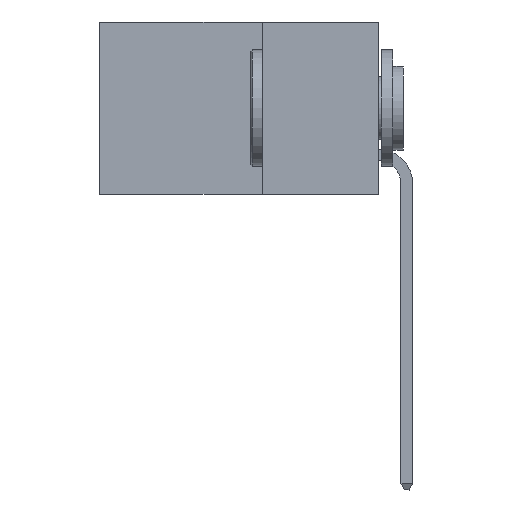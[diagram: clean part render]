
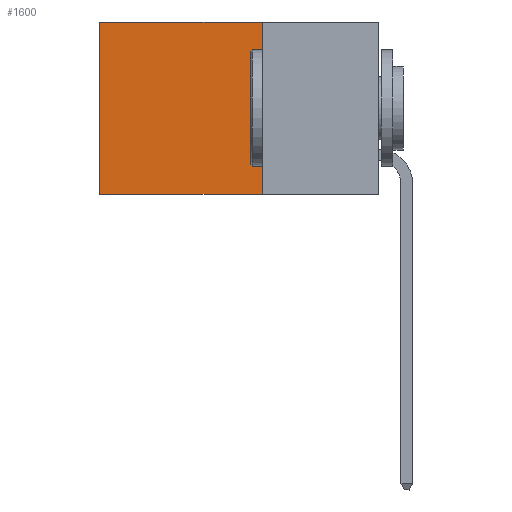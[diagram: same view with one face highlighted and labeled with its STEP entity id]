
A CAD part, left-side view. The second image highlights one B-rep face of the part: STEP entity #1600.
In plain terms, the highlighted planar face has unit normal (-1, 0, 0).
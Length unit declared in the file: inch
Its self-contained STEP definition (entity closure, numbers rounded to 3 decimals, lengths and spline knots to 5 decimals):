
#250 = CARTESIAN_POINT ( 'NONE',  ( 0.298, 0.25, 0. ) ) ;
#431 = AXIS2_PLACEMENT_3D ( 'NONE', #1900, #26840, #19964 ) ;
#1600 = ADVANCED_FACE ( 'NONE', ( #22351 ), #2191, .F. ) ;
#1900 = CARTESIAN_POINT ( 'NONE',  ( 0.298, 0.25, 0. ) ) ;
#2105 = VECTOR ( 'NONE', #18477, 39.37008 ) ;
#2172 = CARTESIAN_POINT ( 'NONE',  ( 0.298, 0.6, 0. ) ) ;
#2191 = PLANE ( 'NONE',  #431 ) ;
#3347 = ORIENTED_EDGE ( 'NONE', *, *, #16645, .F. ) ;
#3802 = CARTESIAN_POINT ( 'NONE',  ( 0.298, 0.25, -0.37 ) ) ;
#3973 = EDGE_CURVE ( 'NONE', #8858, #10029, #18820, .T. ) ;
#4275 = VECTOR ( 'NONE', #25693, 39.37008 ) ;
#5141 = ORIENTED_EDGE ( 'NONE', *, *, #5374, .F. ) ;
#5374 = EDGE_CURVE ( 'NONE', #27201, #7187, #15088, .T. ) ;
#5872 = LINE ( 'NONE', #3802, #24953 ) ;
#6548 = DIRECTION ( 'NONE',  ( 0., 0., -1. ) ) ;
#7187 = VERTEX_POINT ( 'NONE', #27425 ) ;
#7457 = CARTESIAN_POINT ( 'NONE',  ( 0.298, 0.6, 0. ) ) ;
#8858 = VERTEX_POINT ( 'NONE', #2172 ) ;
#9078 = LINE ( 'NONE', #250, #2105 ) ;
#10029 = VERTEX_POINT ( 'NONE', #20120 ) ;
#13866 = EDGE_LOOP ( 'NONE', ( #25352, #3347, #5141, #16098 ) ) ;
#15088 = LINE ( 'NONE', #17914, #23397 ) ;
#15148 = DIRECTION ( 'NONE',  ( 0., 1., 0. ) ) ;
#16063 = EDGE_CURVE ( 'NONE', #27201, #8858, #9078, .T. ) ;
#16098 = ORIENTED_EDGE ( 'NONE', *, *, #16063, .T. ) ;
#16645 = EDGE_CURVE ( 'NONE', #7187, #10029, #5872, .T. ) ;
#17914 = CARTESIAN_POINT ( 'NONE',  ( 0.298, 0.25, 0. ) ) ;
#18477 = DIRECTION ( 'NONE',  ( 0., 1., 0. ) ) ;
#18820 = LINE ( 'NONE', #7457, #4275 ) ;
#19019 = CARTESIAN_POINT ( 'NONE',  ( 0.298, 0.25, 0. ) ) ;
#19964 = DIRECTION ( 'NONE',  ( 0., 0., -1. ) ) ;
#20120 = CARTESIAN_POINT ( 'NONE',  ( 0.298, 0.6, -0.37 ) ) ;
#22351 = FACE_OUTER_BOUND ( 'NONE', #13866, .T. ) ;
#23397 = VECTOR ( 'NONE', #6548, 39.37008 ) ;
#24953 = VECTOR ( 'NONE', #15148, 39.37008 ) ;
#25352 = ORIENTED_EDGE ( 'NONE', *, *, #3973, .T. ) ;
#25693 = DIRECTION ( 'NONE',  ( 0., 0., -1. ) ) ;
#26840 = DIRECTION ( 'NONE',  ( 1., 0., 0. ) ) ;
#27201 = VERTEX_POINT ( 'NONE', #19019 ) ;
#27425 = CARTESIAN_POINT ( 'NONE',  ( 0.298, 0.25, -0.37 ) ) ;
